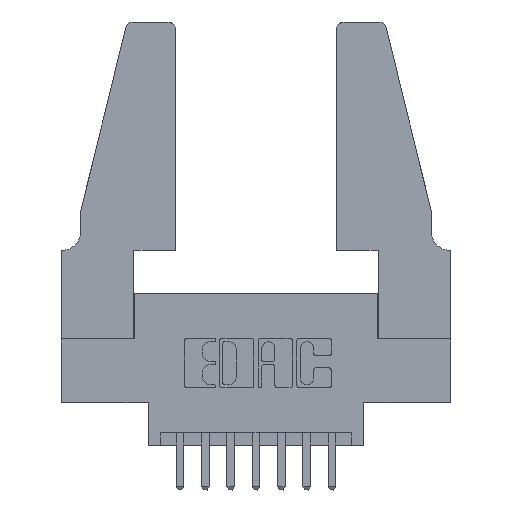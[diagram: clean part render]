
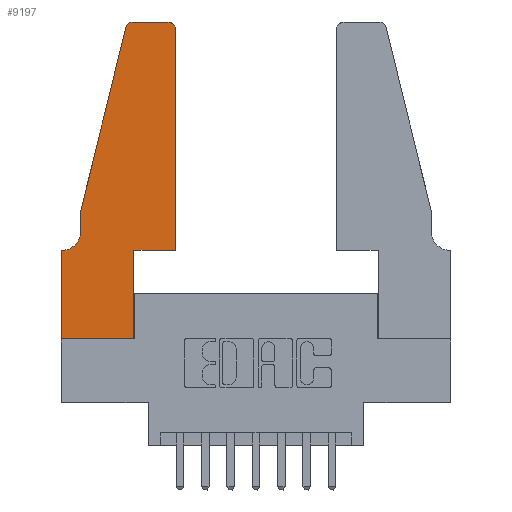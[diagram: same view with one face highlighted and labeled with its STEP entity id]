
A CAD part, top view. The second image highlights one B-rep face of the part: STEP entity #9197.
In plain terms, the highlighted planar face has unit normal (0, 0, 1).
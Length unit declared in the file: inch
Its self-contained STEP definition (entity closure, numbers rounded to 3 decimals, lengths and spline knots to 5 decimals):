
#102 = VECTOR ( 'NONE', #3082, 39.37008 ) ;
#119 = CARTESIAN_POINT ( 'NONE',  ( 0.2865, 0.35, 0.37 ) ) ;
#718 = CARTESIAN_POINT ( 'NONE',  ( 0., 0., 0.37 ) ) ;
#839 = CARTESIAN_POINT ( 'NONE',  ( 0., 0.35, 0.37 ) ) ;
#893 = ORIENTED_EDGE ( 'NONE', *, *, #7593, .T. ) ;
#1165 = CARTESIAN_POINT ( 'NONE',  ( 0., 0., 0.37 ) ) ;
#1205 = CARTESIAN_POINT ( 'NONE',  ( 0.0055, 0.42, 0.37 ) ) ;
#1325 = AXIS2_PLACEMENT_3D ( 'NONE', #2887, #12177, #12002 ) ;
#1845 = DIRECTION ( 'NONE',  ( 0., 0., 1. ) ) ;
#2070 = EDGE_CURVE ( 'NONE', #10418, #9541, #8364, .T. ) ;
#2149 = ORIENTED_EDGE ( 'NONE', *, *, #3983, .T. ) ;
#2203 = ORIENTED_EDGE ( 'NONE', *, *, #10061, .T. ) ;
#2227 = DIRECTION ( 'NONE',  ( -1., 0., 0. ) ) ;
#2887 = CARTESIAN_POINT ( 'NONE',  ( 0.4205, 1.22, 0.37 ) ) ;
#2904 = CARTESIAN_POINT ( 'NONE',  ( 0.4505, 0.35, 0.37 ) ) ;
#2987 = LINE ( 'NONE', #2904, #7584 ) ;
#3082 = DIRECTION ( 'NONE',  ( -0.239, -0.971, 0. ) ) ;
#3203 = LINE ( 'NONE', #12402, #10354 ) ;
#3294 = ORIENTED_EDGE ( 'NONE', *, *, #8754, .T. ) ;
#3311 = CARTESIAN_POINT ( 'NONE',  ( 0.4505, 0.35, 0.37 ) ) ;
#3391 = LINE ( 'NONE', #5041, #102 ) ;
#3848 = VERTEX_POINT ( 'NONE', #3869 ) ;
#3859 = AXIS2_PLACEMENT_3D ( 'NONE', #1205, #8056, #2227 ) ;
#3869 = CARTESIAN_POINT ( 'NONE',  ( 0.0755, 0.42, 0.37 ) ) ;
#3887 = DIRECTION ( 'NONE',  ( 1., 0., 0. ) ) ;
#3983 = EDGE_CURVE ( 'NONE', #5295, #10418, #10286, .T. ) ;
#4017 = CARTESIAN_POINT ( 'NONE',  ( 0.2865, 0.35, 0.37 ) ) ;
#4251 = DIRECTION ( 'NONE',  ( 0., 1., 0. ) ) ;
#4399 = CARTESIAN_POINT ( 'NONE',  ( 0.284, 1.22, 0.37 ) ) ;
#4475 = ORIENTED_EDGE ( 'NONE', *, *, #7922, .T. ) ;
#4484 = EDGE_CURVE ( 'NONE', #10016, #7573, #4821, .T. ) ;
#4821 = LINE ( 'NONE', #4017, #9651 ) ;
#4830 = VECTOR ( 'NONE', #4251, 39.37008 ) ;
#4910 = CARTESIAN_POINT ( 'NONE',  ( 0.0755, 0.5, 0.37 ) ) ;
#5041 = CARTESIAN_POINT ( 'NONE',  ( 0.0755, 0.5, 0.37 ) ) ;
#5295 = VERTEX_POINT ( 'NONE', #3311 ) ;
#5364 = DIRECTION ( 'NONE',  ( 1., 0., 0. ) ) ;
#5494 = VECTOR ( 'NONE', #8556, 39.37008 ) ;
#5594 = CIRCLE ( 'NONE', #12594, 0.03 ) ;
#5619 = ORIENTED_EDGE ( 'NONE', *, *, #7307, .T. ) ;
#5625 = ORIENTED_EDGE ( 'NONE', *, *, #11910, .T. ) ;
#5819 = CARTESIAN_POINT ( 'NONE',  ( 0.4505, 1.22, 0.37 ) ) ;
#5969 = ORIENTED_EDGE ( 'NONE', *, *, #7957, .T. ) ;
#6007 = CARTESIAN_POINT ( 'NONE',  ( 0.0755, 0.35, 0.37 ) ) ;
#6198 = CARTESIAN_POINT ( 'NONE',  ( 0.4505, 0.35, 0.37 ) ) ;
#6222 = EDGE_CURVE ( 'NONE', #11079, #11817, #3391, .T. ) ;
#6277 = CARTESIAN_POINT ( 'NONE',  ( 0.284, 1.25, 0.37 ) ) ;
#6595 = CARTESIAN_POINT ( 'NONE',  ( 0.0755, 0.5, 0.37 ) ) ;
#6711 = PLANE ( 'NONE',  #10110 ) ;
#6757 = CARTESIAN_POINT ( 'NONE',  ( 0.25487, 1.22718, 0.37 ) ) ;
#6986 = DIRECTION ( 'NONE',  ( -1., 0., 0. ) ) ;
#7307 = EDGE_CURVE ( 'NONE', #8731, #10016, #11272, .T. ) ;
#7573 = VERTEX_POINT ( 'NONE', #119 ) ;
#7584 = VECTOR ( 'NONE', #3887, 39.37008 ) ;
#7593 = EDGE_CURVE ( 'NONE', #12225, #8731, #12317, .T. ) ;
#7643 = CIRCLE ( 'NONE', #3859, 0.07 ) ;
#7922 = EDGE_CURVE ( 'NONE', #11817, #3848, #10669, .T. ) ;
#7957 = EDGE_CURVE ( 'NONE', #9541, #11425, #3203, .T. ) ;
#8056 = DIRECTION ( 'NONE',  ( 0., 0., -1. ) ) ;
#8085 = VECTOR ( 'NONE', #11419, 39.37008 ) ;
#8172 = CARTESIAN_POINT ( 'NONE',  ( 0.2865, 0., 0.37 ) ) ;
#8364 = CIRCLE ( 'NONE', #1325, 0.03 ) ;
#8556 = DIRECTION ( 'NONE',  ( 1., 0., 0. ) ) ;
#8649 = DIRECTION ( 'NONE',  ( 1., 0., 0. ) ) ;
#8674 = CARTESIAN_POINT ( 'NONE',  ( 0., 0.35, 0.37 ) ) ;
#8731 = VERTEX_POINT ( 'NONE', #1165 ) ;
#8754 = EDGE_CURVE ( 'NONE', #3848, #9756, #7643, .T. ) ;
#9197 = ADVANCED_FACE ( 'NONE', ( #11841 ), #6711, .T. ) ;
#9541 = VERTEX_POINT ( 'NONE', #12117 ) ;
#9651 = VECTOR ( 'NONE', #10778, 39.37008 ) ;
#9741 = VECTOR ( 'NONE', #11892, 39.37008 ) ;
#9756 = VERTEX_POINT ( 'NONE', #12415 ) ;
#9891 = ORIENTED_EDGE ( 'NONE', *, *, #11765, .T. ) ;
#10016 = VERTEX_POINT ( 'NONE', #8172 ) ;
#10061 = EDGE_CURVE ( 'NONE', #11425, #11079, #5594, .T. ) ;
#10110 = AXIS2_PLACEMENT_3D ( 'NONE', #839, #1845, #8649 ) ;
#10286 = LINE ( 'NONE', #6198, #4830 ) ;
#10354 = VECTOR ( 'NONE', #11465, 39.37008 ) ;
#10418 = VERTEX_POINT ( 'NONE', #5819 ) ;
#10669 = LINE ( 'NONE', #6595, #8085 ) ;
#10778 = DIRECTION ( 'NONE',  ( 0., 1., 0. ) ) ;
#10916 = CARTESIAN_POINT ( 'NONE',  ( 0., 0., 0.37 ) ) ;
#11079 = VERTEX_POINT ( 'NONE', #6757 ) ;
#11186 = DIRECTION ( 'NONE',  ( 0., 0., 1. ) ) ;
#11193 = VECTOR ( 'NONE', #6986, 39.37008 ) ;
#11272 = LINE ( 'NONE', #718, #5494 ) ;
#11419 = DIRECTION ( 'NONE',  ( 0., -1., 0. ) ) ;
#11425 = VERTEX_POINT ( 'NONE', #6277 ) ;
#11449 = ORIENTED_EDGE ( 'NONE', *, *, #2070, .T. ) ;
#11465 = DIRECTION ( 'NONE',  ( -1., 0., 0. ) ) ;
#11712 = ORIENTED_EDGE ( 'NONE', *, *, #4484, .T. ) ;
#11743 = EDGE_LOOP ( 'NONE', ( #5969, #2203, #11853, #4475, #3294, #5625, #893, #5619, #11712, #9891, #2149, #11449 ) ) ;
#11765 = EDGE_CURVE ( 'NONE', #7573, #5295, #2987, .T. ) ;
#11797 = LINE ( 'NONE', #6007, #11193 ) ;
#11817 = VERTEX_POINT ( 'NONE', #4910 ) ;
#11841 = FACE_OUTER_BOUND ( 'NONE', #11743, .T. ) ;
#11853 = ORIENTED_EDGE ( 'NONE', *, *, #6222, .T. ) ;
#11892 = DIRECTION ( 'NONE',  ( 0., -1., 0. ) ) ;
#11910 = EDGE_CURVE ( 'NONE', #9756, #12225, #11797, .T. ) ;
#12002 = DIRECTION ( 'NONE',  ( 1., 0., 0. ) ) ;
#12117 = CARTESIAN_POINT ( 'NONE',  ( 0.4205, 1.25, 0.37 ) ) ;
#12177 = DIRECTION ( 'NONE',  ( 0., 0., 1. ) ) ;
#12225 = VERTEX_POINT ( 'NONE', #8674 ) ;
#12317 = LINE ( 'NONE', #10916, #9741 ) ;
#12402 = CARTESIAN_POINT ( 'NONE',  ( 0.2605, 1.25, 0.37 ) ) ;
#12415 = CARTESIAN_POINT ( 'NONE',  ( 0.0055, 0.35, 0.37 ) ) ;
#12594 = AXIS2_PLACEMENT_3D ( 'NONE', #4399, #11186, #5364 ) ;
